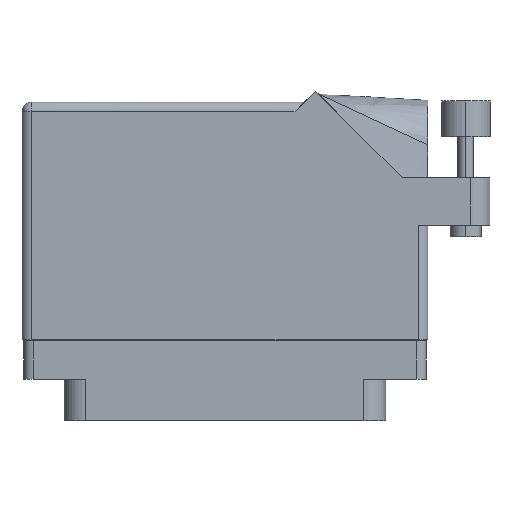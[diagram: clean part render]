
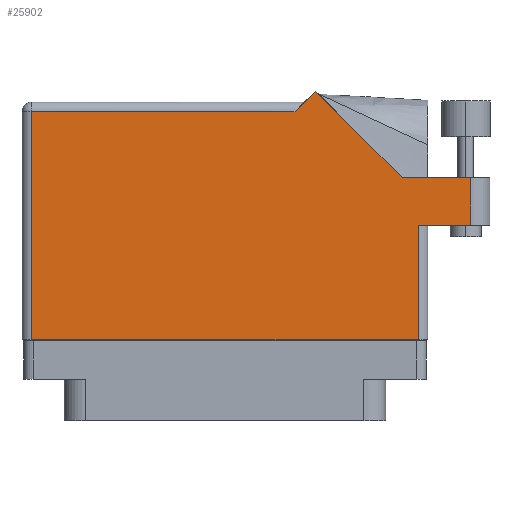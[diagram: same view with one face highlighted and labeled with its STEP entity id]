
A CAD part, front view. The second image highlights one B-rep face of the part: STEP entity #25902.
In plain terms, the highlighted face is planar.
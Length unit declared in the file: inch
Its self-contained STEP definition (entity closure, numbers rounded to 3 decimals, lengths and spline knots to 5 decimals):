
#273 = CARTESIAN_POINT ( 'NONE',  ( 1.581, 0.944, 0.455 ) ) ;
#505 = DIRECTION ( 'NONE',  ( -0.707, 0.707, 0. ) ) ;
#1689 = ORIENTED_EDGE ( 'NONE', *, *, #8675, .T. ) ;
#2304 = DIRECTION ( 'NONE',  ( -1., 0., 0. ) ) ;
#2603 = DIRECTION ( 'NONE',  ( 1., 0., 0. ) ) ;
#4201 = VECTOR ( 'NONE', #2603, 39.37008 ) ;
#4343 = ORIENTED_EDGE ( 'NONE', *, *, #30986, .T. ) ;
#4724 = DIRECTION ( 'NONE',  ( 0., 1., 0. ) ) ;
#5794 = CARTESIAN_POINT ( 'NONE',  ( 0.513, 1.43, 0.455 ) ) ;
#6677 = EDGE_CURVE ( 'NONE', #19362, #44409, #37280, .T. ) ;
#6841 = ORIENTED_EDGE ( 'NONE', *, *, #9153, .T. ) ;
#6939 = CARTESIAN_POINT ( 'NONE',  ( 0.58371, 1.50071, 0.455 ) ) ;
#7369 = VERTEX_POINT ( 'NONE', #273 ) ;
#7972 = VECTOR ( 'NONE', #2304, 39.37008 ) ;
#8067 = CARTESIAN_POINT ( 'NONE',  ( -1.244, -0.1, 0.455 ) ) ;
#8675 = EDGE_CURVE ( 'NONE', #10758, #43096, #16875, .T. ) ;
#8950 = CARTESIAN_POINT ( 'NONE',  ( -1.306, 1.368, 0.455 ) ) ;
#9153 = EDGE_CURVE ( 'NONE', #45398, #46475, #43182, .T. ) ;
#9319 = CARTESIAN_POINT ( 'NONE',  ( 0.451, 1.368, 0.455 ) ) ;
#9590 = CARTESIAN_POINT ( 'NONE',  ( -1.306, 1.43, 0.455 ) ) ;
#10325 = EDGE_CURVE ( 'NONE', #36753, #45398, #28034, .T. ) ;
#10330 = CARTESIAN_POINT ( 'NONE',  ( 1.244, 0.637, 0.455 ) ) ;
#10758 = VERTEX_POINT ( 'NONE', #10330 ) ;
#11262 = ORIENTED_EDGE ( 'NONE', *, *, #34868, .T. ) ;
#11895 = LINE ( 'NONE', #41240, #14183 ) ;
#12195 = CARTESIAN_POINT ( 'NONE',  ( 1.14042, 0.944, 0.455 ) ) ;
#12565 = VECTOR ( 'NONE', #30395, 39.37008 ) ;
#12567 = ORIENTED_EDGE ( 'NONE', *, *, #10325, .T. ) ;
#13716 = DIRECTION ( 'NONE',  ( -1., 0., 0. ) ) ;
#13744 = DIRECTION ( 'NONE',  ( -0.707, -0.707, 0. ) ) ;
#13893 = DIRECTION ( 'NONE',  ( 0., -1., 0. ) ) ;
#14077 = CARTESIAN_POINT ( 'NONE',  ( 1.244, -0.1, 0.455 ) ) ;
#14183 = VECTOR ( 'NONE', #4724, 39.37008 ) ;
#14837 = LINE ( 'NONE', #17033, #7972 ) ;
#15363 = CARTESIAN_POINT ( 'NONE',  ( 1.581, 0.637, 0.455 ) ) ;
#15685 = DIRECTION ( 'NONE',  ( -1., 0., 0. ) ) ;
#16875 = LINE ( 'NONE', #18262, #32881 ) ;
#17033 = CARTESIAN_POINT ( 'NONE',  ( 1.706, 0.944, 0.455 ) ) ;
#18262 = CARTESIAN_POINT ( 'NONE',  ( 1.306, 0.637, 0.455 ) ) ;
#18865 = LINE ( 'NONE', #37652, #12565 ) ;
#19362 = VERTEX_POINT ( 'NONE', #6939 ) ;
#21239 = EDGE_CURVE ( 'NONE', #7369, #30548, #14837, .T. ) ;
#21314 = ORIENTED_EDGE ( 'NONE', *, *, #21239, .T. ) ;
#22275 = CARTESIAN_POINT ( 'NONE',  ( 1.14042, 0.944, 0.455 ) ) ;
#25020 = CARTESIAN_POINT ( 'NONE',  ( -1.306, -0.1, 0.455 ) ) ;
#25902 = ADVANCED_FACE ( 'NONE', ( #45307 ), #35020, .F. ) ;
#26730 = AXIS2_PLACEMENT_3D ( 'NONE', #9590, #27938, #13716 ) ;
#27219 = EDGE_CURVE ( 'NONE', #43096, #7369, #18865, .T. ) ;
#27267 = CARTESIAN_POINT ( 'NONE',  ( -1.244, 1.368, 0.455 ) ) ;
#27938 = DIRECTION ( 'NONE',  ( 0., 0., -1. ) ) ;
#28034 = LINE ( 'NONE', #46573, #33219 ) ;
#28603 = ORIENTED_EDGE ( 'NONE', *, *, #46662, .T. ) ;
#30395 = DIRECTION ( 'NONE',  ( 0., 1., 0. ) ) ;
#30548 = VERTEX_POINT ( 'NONE', #12195 ) ;
#30986 = EDGE_CURVE ( 'NONE', #44409, #36753, #36281, .T. ) ;
#31635 = VECTOR ( 'NONE', #15685, 39.37008 ) ;
#32881 = VECTOR ( 'NONE', #40578, 39.37008 ) ;
#33219 = VECTOR ( 'NONE', #13893, 39.37008 ) ;
#34647 = LINE ( 'NONE', #22275, #47261 ) ;
#34868 = EDGE_CURVE ( 'NONE', #46475, #10758, #11895, .T. ) ;
#35020 = PLANE ( 'NONE',  #26730 ) ;
#36281 = LINE ( 'NONE', #8950, #31635 ) ;
#36739 = ORIENTED_EDGE ( 'NONE', *, *, #27219, .T. ) ;
#36753 = VERTEX_POINT ( 'NONE', #27267 ) ;
#37280 = LINE ( 'NONE', #5794, #45887 ) ;
#37652 = CARTESIAN_POINT ( 'NONE',  ( 1.581, 0.944, 0.455 ) ) ;
#40578 = DIRECTION ( 'NONE',  ( 1., 0., 0. ) ) ;
#41240 = CARTESIAN_POINT ( 'NONE',  ( 1.244, 0.637, 0.455 ) ) ;
#42936 = EDGE_LOOP ( 'NONE', ( #1689, #36739, #21314, #28603, #46936, #4343, #12567, #6841, #11262 ) ) ;
#43096 = VERTEX_POINT ( 'NONE', #15363 ) ;
#43182 = LINE ( 'NONE', #25020, #4201 ) ;
#44409 = VERTEX_POINT ( 'NONE', #9319 ) ;
#45307 = FACE_OUTER_BOUND ( 'NONE', #42936, .T. ) ;
#45398 = VERTEX_POINT ( 'NONE', #8067 ) ;
#45887 = VECTOR ( 'NONE', #13744, 39.37008 ) ;
#46475 = VERTEX_POINT ( 'NONE', #14077 ) ;
#46573 = CARTESIAN_POINT ( 'NONE',  ( -1.244, -0.1, 0.455 ) ) ;
#46662 = EDGE_CURVE ( 'NONE', #30548, #19362, #34647, .T. ) ;
#46936 = ORIENTED_EDGE ( 'NONE', *, *, #6677, .T. ) ;
#47261 = VECTOR ( 'NONE', #505, 39.37008 ) ;
